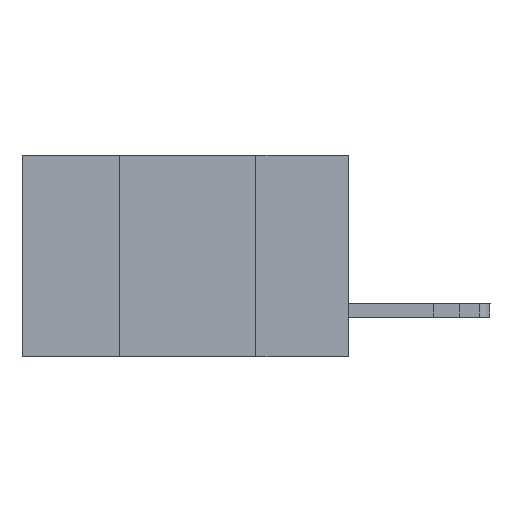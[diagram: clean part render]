
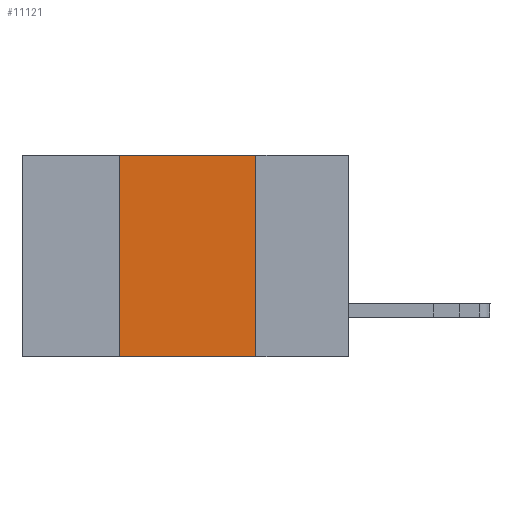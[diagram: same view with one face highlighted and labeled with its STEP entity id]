
A CAD part, left-side view. The second image highlights one B-rep face of the part: STEP entity #11121.
In plain terms, the highlighted planar face has unit normal (-1, 0, 0).
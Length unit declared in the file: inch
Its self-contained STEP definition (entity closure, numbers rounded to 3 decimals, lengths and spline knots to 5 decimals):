
#42 = ORIENTED_EDGE ( 'NONE', *, *, #12816, .F. ) ;
#179 = VECTOR ( 'NONE', #646, 39.37008 ) ;
#425 = CARTESIAN_POINT ( 'NONE',  ( 0., 0.17, -0.37 ) ) ;
#646 = DIRECTION ( 'NONE',  ( 0., 0., -1. ) ) ;
#2759 = LINE ( 'NONE', #15529, #3195 ) ;
#2971 = DIRECTION ( 'NONE',  ( 0., 0., -1. ) ) ;
#3195 = VECTOR ( 'NONE', #4082, 39.37008 ) ;
#3844 = EDGE_LOOP ( 'NONE', ( #42, #11253, #6970, #14066 ) ) ;
#4082 = DIRECTION ( 'NONE',  ( 0., 0., 1. ) ) ;
#4451 = FACE_OUTER_BOUND ( 'NONE', #3844, .T. ) ;
#4501 = VERTEX_POINT ( 'NONE', #13574 ) ;
#4551 = CARTESIAN_POINT ( 'NONE',  ( 0., 0.6, 0. ) ) ;
#5660 = VERTEX_POINT ( 'NONE', #425 ) ;
#6172 = EDGE_CURVE ( 'NONE', #13215, #5660, #15394, .T. ) ;
#6970 = ORIENTED_EDGE ( 'NONE', *, *, #8177, .F. ) ;
#7468 = DIRECTION ( 'NONE',  ( 0., -1., 0. ) ) ;
#7978 = CARTESIAN_POINT ( 'NONE',  ( 0., 0.17, -0.37 ) ) ;
#8041 = LINE ( 'NONE', #7978, #179 ) ;
#8177 = EDGE_CURVE ( 'NONE', #13215, #4501, #2759, .T. ) ;
#9153 = EDGE_CURVE ( 'NONE', #4501, #11594, #14092, .T. ) ;
#10197 = CARTESIAN_POINT ( 'NONE',  ( 0., 0.6, 0. ) ) ;
#10403 = VECTOR ( 'NONE', #7468, 39.37008 ) ;
#11121 = ADVANCED_FACE ( 'NONE', ( #4451 ), #18449, .F. ) ;
#11253 = ORIENTED_EDGE ( 'NONE', *, *, #9153, .F. ) ;
#11588 = DIRECTION ( 'NONE',  ( 1., 0., 0. ) ) ;
#11594 = VERTEX_POINT ( 'NONE', #12733 ) ;
#11707 = VECTOR ( 'NONE', #16432, 39.37008 ) ;
#12733 = CARTESIAN_POINT ( 'NONE',  ( 0., 0.17, 0. ) ) ;
#12816 = EDGE_CURVE ( 'NONE', #11594, #5660, #8041, .T. ) ;
#13215 = VERTEX_POINT ( 'NONE', #17200 ) ;
#13574 = CARTESIAN_POINT ( 'NONE',  ( 0., 0.42, 0. ) ) ;
#14066 = ORIENTED_EDGE ( 'NONE', *, *, #6172, .T. ) ;
#14092 = LINE ( 'NONE', #4551, #10403 ) ;
#15394 = LINE ( 'NONE', #16652, #11707 ) ;
#15529 = CARTESIAN_POINT ( 'NONE',  ( 0., 0.42, -0.37 ) ) ;
#15912 = AXIS2_PLACEMENT_3D ( 'NONE', #10197, #11588, #2971 ) ;
#16432 = DIRECTION ( 'NONE',  ( 0., -1., 0. ) ) ;
#16652 = CARTESIAN_POINT ( 'NONE',  ( 0., 0.6, -0.37 ) ) ;
#17200 = CARTESIAN_POINT ( 'NONE',  ( 0., 0.42, -0.37 ) ) ;
#18449 = PLANE ( 'NONE',  #15912 ) ;
